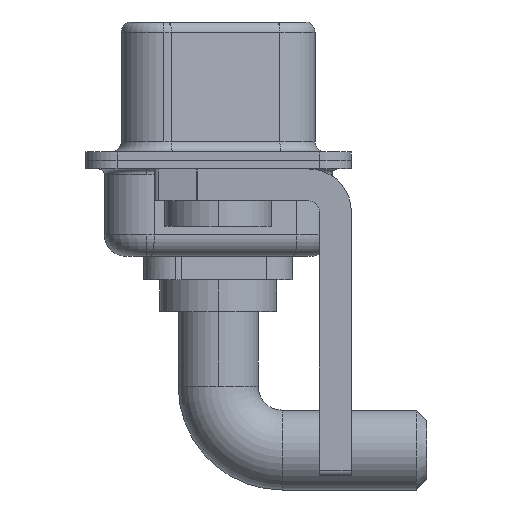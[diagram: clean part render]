
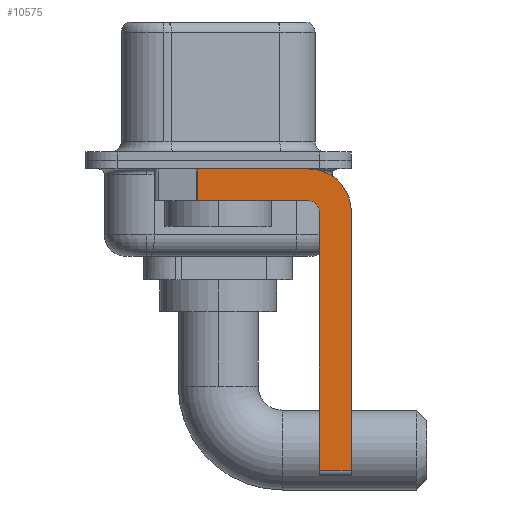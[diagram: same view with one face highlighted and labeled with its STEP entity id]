
A CAD part, left-side view. The second image highlights one B-rep face of the part: STEP entity #10575.
In plain terms, the highlighted planar face has unit normal (-1, 0, 0).
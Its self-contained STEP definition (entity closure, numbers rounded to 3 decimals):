
#1154 = FACE_OUTER_BOUND ( 'NONE', #6293, .T. ) ;
#1473 = EDGE_CURVE ( 'NONE', #2033, #16039, #14730, .T. ) ;
#1652 = VECTOR ( 'NONE', #2876, 1000. ) ;
#1667 = CARTESIAN_POINT ( 'NONE',  ( -2.9, -4.25, -1.9 ) ) ;
#1768 = CARTESIAN_POINT ( 'NONE',  ( -2.9, -4.75, -14.55 ) ) ;
#1885 = ORIENTED_EDGE ( 'NONE', *, *, #15310, .F. ) ;
#1971 = LINE ( 'NONE', #11924, #8291 ) ;
#2033 = VERTEX_POINT ( 'NONE', #10496 ) ;
#2436 = PLANE ( 'NONE',  #3451 ) ;
#2631 = CARTESIAN_POINT ( 'NONE',  ( -2.9, 0.978, -1.9 ) ) ;
#2782 = VERTEX_POINT ( 'NONE', #12065 ) ;
#2876 = DIRECTION ( 'NONE',  ( 0., 0., -1. ) ) ;
#3098 = VERTEX_POINT ( 'NONE', #1768 ) ;
#3451 = AXIS2_PLACEMENT_3D ( 'NONE', #3895, #15449, #5099 ) ;
#3895 = CARTESIAN_POINT ( 'NONE',  ( -2.9, -4.25, -2.4 ) ) ;
#4007 = CARTESIAN_POINT ( 'NONE',  ( -2.9, -4.25, -14.55 ) ) ;
#4153 = DIRECTION ( 'NONE',  ( 0., 0., 1. ) ) ;
#4673 = LINE ( 'NONE', #8476, #12632 ) ;
#4742 = ORIENTED_EDGE ( 'NONE', *, *, #5793, .T. ) ;
#4976 = CARTESIAN_POINT ( 'NONE',  ( -2.9, -4.75, -2.4 ) ) ;
#5099 = DIRECTION ( 'NONE',  ( 0., 0., -1. ) ) ;
#5698 = LINE ( 'NONE', #8206, #10073 ) ;
#5777 = DIRECTION ( 'NONE',  ( 0., 0., 1. ) ) ;
#5793 = EDGE_CURVE ( 'NONE', #2782, #13010, #9017, .T. ) ;
#6289 = EDGE_CURVE ( 'NONE', #10340, #13010, #1971, .T. ) ;
#6293 = EDGE_LOOP ( 'NONE', ( #9950, #4742, #6410, #1885, #10710, #15710, #9657, #16511 ) ) ;
#6320 = VERTEX_POINT ( 'NONE', #14894 ) ;
#6410 = ORIENTED_EDGE ( 'NONE', *, *, #6289, .F. ) ;
#7318 = AXIS2_PLACEMENT_3D ( 'NONE', #11492, #15596, #12782 ) ;
#7325 = CARTESIAN_POINT ( 'NONE',  ( -2.9, -4.25, -2.4 ) ) ;
#8206 = CARTESIAN_POINT ( 'NONE',  ( -2.9, -4.75, -14.8 ) ) ;
#8291 = VECTOR ( 'NONE', #14972, 1000. ) ;
#8476 = CARTESIAN_POINT ( 'NONE',  ( -2.9, -6.25, -2.4 ) ) ;
#8569 = DIRECTION ( 'NONE',  ( 0., 0., -1. ) ) ;
#9017 = LINE ( 'NONE', #13229, #1652 ) ;
#9030 = VECTOR ( 'NONE', #12032, 1000. ) ;
#9255 = EDGE_CURVE ( 'NONE', #2782, #2033, #15925, .T. ) ;
#9657 = ORIENTED_EDGE ( 'NONE', *, *, #14890, .F. ) ;
#9950 = ORIENTED_EDGE ( 'NONE', *, *, #9255, .F. ) ;
#10073 = VECTOR ( 'NONE', #4153, 1000. ) ;
#10340 = VERTEX_POINT ( 'NONE', #1667 ) ;
#10496 = CARTESIAN_POINT ( 'NONE',  ( -2.9, -4.25, -0.4 ) ) ;
#10575 = ADVANCED_FACE ( 'NONE', ( #1154 ), #2436, .F. ) ;
#10710 = ORIENTED_EDGE ( 'NONE', *, *, #10773, .F. ) ;
#10773 = EDGE_CURVE ( 'NONE', #3098, #12816, #5698, .T. ) ;
#11492 = CARTESIAN_POINT ( 'NONE',  ( -2.9, -4.25, -2.4 ) ) ;
#11543 = AXIS2_PLACEMENT_3D ( 'NONE', #7325, #12595, #5777 ) ;
#11924 = CARTESIAN_POINT ( 'NONE',  ( -2.9, -4.25, -1.9 ) ) ;
#12032 = DIRECTION ( 'NONE',  ( 0., -1., 0. ) ) ;
#12065 = CARTESIAN_POINT ( 'NONE',  ( -2.9, 0.978, -0.4 ) ) ;
#12119 = LINE ( 'NONE', #4007, #9030 ) ;
#12595 = DIRECTION ( 'NONE',  ( -1., 0., 0. ) ) ;
#12611 = EDGE_CURVE ( 'NONE', #3098, #6320, #12119, .T. ) ;
#12632 = VECTOR ( 'NONE', #8569, 1000. ) ;
#12782 = DIRECTION ( 'NONE',  ( 0., 0., -1. ) ) ;
#12816 = VERTEX_POINT ( 'NONE', #4976 ) ;
#13010 = VERTEX_POINT ( 'NONE', #2631 ) ;
#13229 = CARTESIAN_POINT ( 'NONE',  ( -2.9, 0.978, -1.9 ) ) ;
#13550 = DIRECTION ( 'NONE',  ( 0., -1., 0. ) ) ;
#14009 = CIRCLE ( 'NONE', #11543, 0.5 ) ;
#14571 = CARTESIAN_POINT ( 'NONE',  ( -2.9, 3., -0.4 ) ) ;
#14730 = CIRCLE ( 'NONE', #7318, 2. ) ;
#14890 = EDGE_CURVE ( 'NONE', #16039, #6320, #4673, .T. ) ;
#14894 = CARTESIAN_POINT ( 'NONE',  ( -2.9, -6.25, -14.55 ) ) ;
#14972 = DIRECTION ( 'NONE',  ( 0., 1., 0. ) ) ;
#15310 = EDGE_CURVE ( 'NONE', #12816, #10340, #14009, .T. ) ;
#15449 = DIRECTION ( 'NONE',  ( 1., 0., 0. ) ) ;
#15596 = DIRECTION ( 'NONE',  ( 1., 0., 0. ) ) ;
#15710 = ORIENTED_EDGE ( 'NONE', *, *, #12611, .T. ) ;
#15925 = LINE ( 'NONE', #14571, #16065 ) ;
#16039 = VERTEX_POINT ( 'NONE', #16046 ) ;
#16046 = CARTESIAN_POINT ( 'NONE',  ( -2.9, -6.25, -2.4 ) ) ;
#16065 = VECTOR ( 'NONE', #13550, 1000. ) ;
#16511 = ORIENTED_EDGE ( 'NONE', *, *, #1473, .F. ) ;
